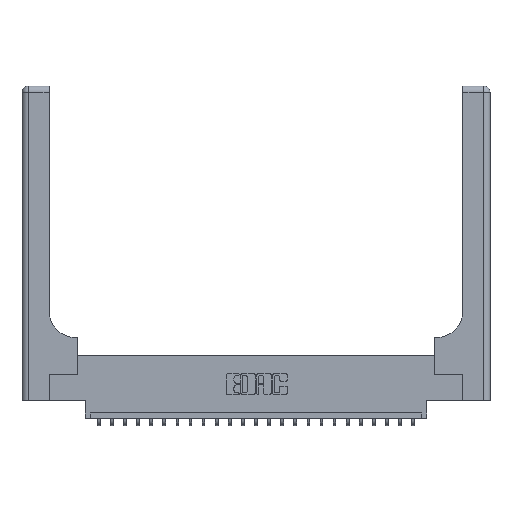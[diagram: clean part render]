
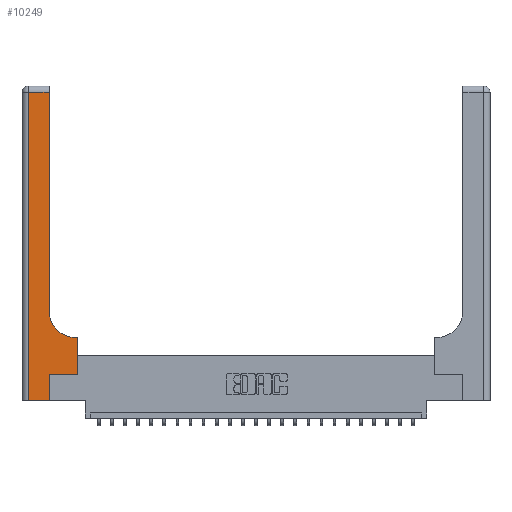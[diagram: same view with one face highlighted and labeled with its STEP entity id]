
A CAD part, top view. The second image highlights one B-rep face of the part: STEP entity #10249.
In plain terms, the highlighted planar face has unit normal (0, 0, 1).
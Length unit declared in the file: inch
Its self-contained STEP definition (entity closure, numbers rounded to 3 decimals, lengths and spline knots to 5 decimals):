
#138 = LINE ( 'NONE', #11142, #15408 ) ;
#537 = CARTESIAN_POINT ( 'NONE',  ( 0., 0., 0.37 ) ) ;
#566 = DIRECTION ( 'NONE',  ( 0., 0., -1. ) ) ;
#958 = ORIENTED_EDGE ( 'NONE', *, *, #17076, .T. ) ;
#1036 = EDGE_CURVE ( 'NONE', #12922, #23296, #8804, .T. ) ;
#1184 = CARTESIAN_POINT ( 'NONE',  ( 0.06, 3., 0.37 ) ) ;
#1376 = DIRECTION ( 'NONE',  ( 0., 0., -1. ) ) ;
#1515 = VECTOR ( 'NONE', #3900, 39.37008 ) ;
#1981 = EDGE_CURVE ( 'NONE', #6069, #21862, #8606, .T. ) ;
#2332 = DIRECTION ( 'NONE',  ( -1., 0., 0. ) ) ;
#2430 = ORIENTED_EDGE ( 'NONE', *, *, #20838, .T. ) ;
#2612 = EDGE_CURVE ( 'NONE', #21862, #12922, #13230, .T. ) ;
#3157 = CARTESIAN_POINT ( 'NONE',  ( 0., 3., 0.37 ) ) ;
#3900 = DIRECTION ( 'NONE',  ( 1., 0., 0. ) ) ;
#4128 = CARTESIAN_POINT ( 'NONE',  ( 0.26, 0.6, 0.37 ) ) ;
#4241 = DIRECTION ( 'NONE',  ( 1., 0., 0. ) ) ;
#5114 = CARTESIAN_POINT ( 'NONE',  ( 0.265, 0.25, 0.37 ) ) ;
#5192 = VECTOR ( 'NONE', #4241, 39.37008 ) ;
#5515 = LINE ( 'NONE', #9459, #5554 ) ;
#5554 = VECTOR ( 'NONE', #16516, 39.37008 ) ;
#6069 = VERTEX_POINT ( 'NONE', #9391 ) ;
#6450 = DIRECTION ( 'NONE',  ( 0., 1., 0. ) ) ;
#7338 = VECTOR ( 'NONE', #6450, 39.37008 ) ;
#7502 = CARTESIAN_POINT ( 'NONE',  ( 0.26, 2.94, 0.37 ) ) ;
#8089 = EDGE_CURVE ( 'NONE', #21563, #9036, #14576, .T. ) ;
#8529 = ORIENTED_EDGE ( 'NONE', *, *, #1036, .T. ) ;
#8606 = LINE ( 'NONE', #23190, #7338 ) ;
#8804 = CIRCLE ( 'NONE', #22164, 0.25 ) ;
#9036 = VERTEX_POINT ( 'NONE', #13171 ) ;
#9248 = EDGE_CURVE ( 'NONE', #9036, #17238, #21398, .T. ) ;
#9391 = CARTESIAN_POINT ( 'NONE',  ( 0.528, 0.25, 0.37 ) ) ;
#9459 = CARTESIAN_POINT ( 'NONE',  ( 0.265, 0., 0.37 ) ) ;
#9752 = AXIS2_PLACEMENT_3D ( 'NONE', #3157, #1376, #15975 ) ;
#9778 = DIRECTION ( 'NONE',  ( 1., 0., 0. ) ) ;
#10106 = CARTESIAN_POINT ( 'NONE',  ( 0.06, 0., 0.37 ) ) ;
#10233 = CARTESIAN_POINT ( 'NONE',  ( 0.528, 0.6, 0.37 ) ) ;
#10249 = ADVANCED_FACE ( 'NONE', ( #12253 ), #19557, .F. ) ;
#11142 = CARTESIAN_POINT ( 'NONE',  ( 0.26, 3., 0.37 ) ) ;
#11235 = VECTOR ( 'NONE', #12309, 39.37008 ) ;
#11597 = ORIENTED_EDGE ( 'NONE', *, *, #1981, .T. ) ;
#11662 = VERTEX_POINT ( 'NONE', #11884 ) ;
#11742 = EDGE_CURVE ( 'NONE', #19168, #11662, #5515, .T. ) ;
#11850 = ORIENTED_EDGE ( 'NONE', *, *, #12688, .T. ) ;
#11884 = CARTESIAN_POINT ( 'NONE',  ( 0.265, 0.25, 0.37 ) ) ;
#12253 = FACE_OUTER_BOUND ( 'NONE', #16434, .T. ) ;
#12309 = DIRECTION ( 'NONE',  ( 0., -1., 0. ) ) ;
#12688 = EDGE_CURVE ( 'NONE', #17238, #19168, #13688, .T. ) ;
#12922 = VERTEX_POINT ( 'NONE', #19432 ) ;
#13171 = CARTESIAN_POINT ( 'NONE',  ( 0.06, 2.94, 0.37 ) ) ;
#13230 = LINE ( 'NONE', #4128, #20381 ) ;
#13688 = LINE ( 'NONE', #537, #5192 ) ;
#13944 = ORIENTED_EDGE ( 'NONE', *, *, #2612, .T. ) ;
#14576 = LINE ( 'NONE', #18178, #18850 ) ;
#14616 = DIRECTION ( 'NONE',  ( 0., 1., 0. ) ) ;
#15408 = VECTOR ( 'NONE', #14616, 39.37008 ) ;
#15975 = DIRECTION ( 'NONE',  ( -1., 0., 0. ) ) ;
#16027 = DIRECTION ( 'NONE',  ( -1., 0., 0. ) ) ;
#16434 = EDGE_LOOP ( 'NONE', ( #2430, #20189, #18055, #11850, #20979, #958, #11597, #13944, #8529 ) ) ;
#16516 = DIRECTION ( 'NONE',  ( 0., 1., 0. ) ) ;
#17076 = EDGE_CURVE ( 'NONE', #11662, #6069, #21500, .T. ) ;
#17238 = VERTEX_POINT ( 'NONE', #10106 ) ;
#18055 = ORIENTED_EDGE ( 'NONE', *, *, #9248, .T. ) ;
#18178 = CARTESIAN_POINT ( 'NONE',  ( 0., 2.94, 0.37 ) ) ;
#18850 = VECTOR ( 'NONE', #16027, 39.37008 ) ;
#19168 = VERTEX_POINT ( 'NONE', #22287 ) ;
#19432 = CARTESIAN_POINT ( 'NONE',  ( 0.51, 0.6, 0.37 ) ) ;
#19557 = PLANE ( 'NONE',  #9752 ) ;
#20189 = ORIENTED_EDGE ( 'NONE', *, *, #8089, .T. ) ;
#20381 = VECTOR ( 'NONE', #2332, 39.37008 ) ;
#20414 = CARTESIAN_POINT ( 'NONE',  ( 0.26, 0.85, 0.37 ) ) ;
#20838 = EDGE_CURVE ( 'NONE', #23296, #21563, #138, .T. ) ;
#20979 = ORIENTED_EDGE ( 'NONE', *, *, #11742, .T. ) ;
#21398 = LINE ( 'NONE', #1184, #11235 ) ;
#21500 = LINE ( 'NONE', #5114, #1515 ) ;
#21563 = VERTEX_POINT ( 'NONE', #7502 ) ;
#21862 = VERTEX_POINT ( 'NONE', #10233 ) ;
#22164 = AXIS2_PLACEMENT_3D ( 'NONE', #22452, #566, #9778 ) ;
#22287 = CARTESIAN_POINT ( 'NONE',  ( 0.265, 0., 0.37 ) ) ;
#22452 = CARTESIAN_POINT ( 'NONE',  ( 0.51, 0.85, 0.37 ) ) ;
#23190 = CARTESIAN_POINT ( 'NONE',  ( 0.528, 0.25, 0.37 ) ) ;
#23296 = VERTEX_POINT ( 'NONE', #20414 ) ;
